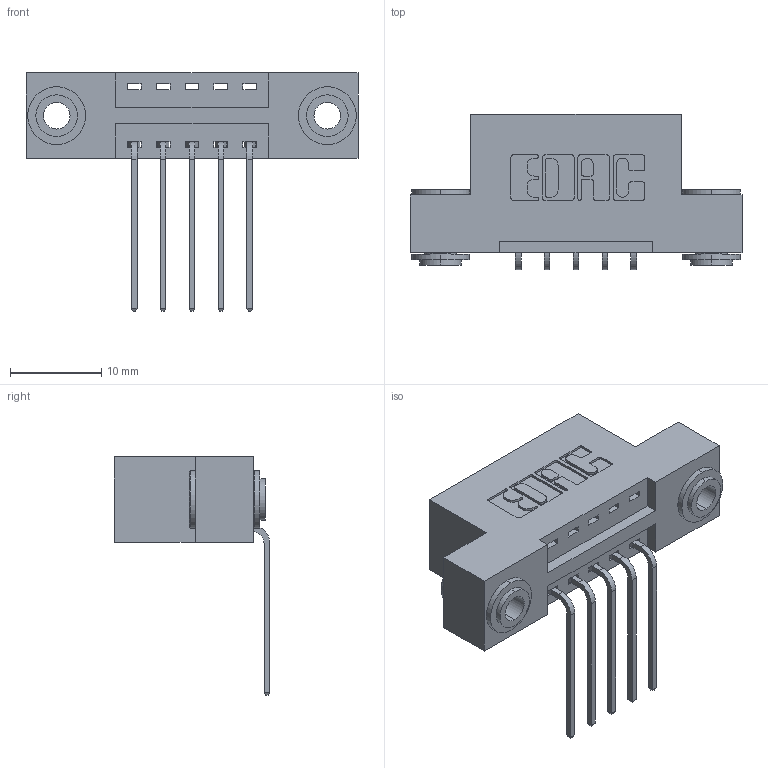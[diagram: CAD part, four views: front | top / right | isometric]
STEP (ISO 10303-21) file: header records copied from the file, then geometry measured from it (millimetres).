
FILE_DESCRIPTION (( 'STEP AP203' ), '1' );
FILE_NAME ('396-005-559-103.STEP', '2018-08-30T22:29:48', ( '' ), ( '' ), 'SwSTEP 2.0', 'SolidWorks 2016', '' );
FILE_SCHEMA (( 'CONFIG_CONTROL_DESIGN' ));
Length unit declared in the file: inch
Products named in the file (4): 346 Part_Flush Mounting Lugs - 0.156 Dia-TH; 345-292-001_558 559 Tail - 1; 345-250-002_345-250-002-102; 396-005-559-103
Assembly tree (8 placements, depth 2):
  396-005-559-103
    346 Part_Flush Mounting Lugs - 0.156 Dia-TH
    345-292-001_558 559 Tail - 1  x5
    345-250-002_345-250-002-102  x2
Bounding box: 36.45 x 17.08 x 26.16 mm (x, y, z)
Volume: 3270.1 mm3; surface area: 4006.5 mm2
Topology: 8 solids, 8 shells, 460 faces, 1315 edges, 866 vertices
Faces by surface type: plane 296, cylinder 156, cone 8
Entity records: 8818 total; most frequent: CARTESIAN_POINT 1502, ORIENTED_EDGE 1434, DIRECTION 1401, EDGE_CURVE 717, LINE 541, VECTOR 541, VERTEX_POINT 474, AXIS2_PLACEMENT_3D 430
